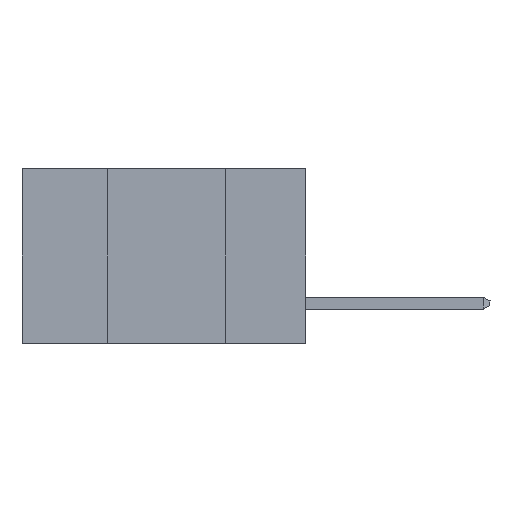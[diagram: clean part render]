
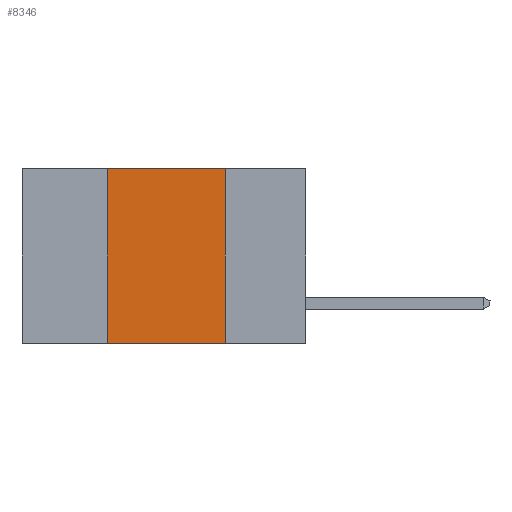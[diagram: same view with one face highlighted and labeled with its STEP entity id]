
A CAD part, left-side view. The second image highlights one B-rep face of the part: STEP entity #8346.
In plain terms, the highlighted planar face has unit normal (-1, 0, 0).
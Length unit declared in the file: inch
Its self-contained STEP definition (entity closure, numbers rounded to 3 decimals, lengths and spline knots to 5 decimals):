
#770 = VERTEX_POINT ( 'NONE', #22254 ) ;
#1752 = CARTESIAN_POINT ( 'NONE',  ( 0., 0.6, 0. ) ) ;
#2187 = VECTOR ( 'NONE', #15263, 39.37008 ) ;
#2382 = CARTESIAN_POINT ( 'NONE',  ( 0., 0.17, -0.37 ) ) ;
#3071 = EDGE_CURVE ( 'NONE', #770, #21164, #15459, .T. ) ;
#3164 = LINE ( 'NONE', #7046, #21861 ) ;
#3831 = ORIENTED_EDGE ( 'NONE', *, *, #11643, .F. ) ;
#4577 = AXIS2_PLACEMENT_3D ( 'NONE', #14930, #9579, #7918 ) ;
#7046 = CARTESIAN_POINT ( 'NONE',  ( 0., 0.42, 0. ) ) ;
#7918 = DIRECTION ( 'NONE',  ( 0., 0., -1. ) ) ;
#7944 = EDGE_LOOP ( 'NONE', ( #8499, #13922, #3831, #9128 ) ) ;
#8346 = ADVANCED_FACE ( 'NONE', ( #8992 ), #20260, .F. ) ;
#8499 = ORIENTED_EDGE ( 'NONE', *, *, #3071, .F. ) ;
#8992 = FACE_OUTER_BOUND ( 'NONE', #7944, .T. ) ;
#9128 = ORIENTED_EDGE ( 'NONE', *, *, #11788, .T. ) ;
#9579 = DIRECTION ( 'NONE',  ( 1., 0., 0. ) ) ;
#9797 = VERTEX_POINT ( 'NONE', #14344 ) ;
#10077 = CARTESIAN_POINT ( 'NONE',  ( 0., 0.17, 0. ) ) ;
#10163 = VECTOR ( 'NONE', #10986, 39.37008 ) ;
#10249 = VERTEX_POINT ( 'NONE', #18871 ) ;
#10726 = LINE ( 'NONE', #1752, #10163 ) ;
#10986 = DIRECTION ( 'NONE',  ( 0., -1., 0. ) ) ;
#11206 = CARTESIAN_POINT ( 'NONE',  ( 0., 0.6, -0.37 ) ) ;
#11643 = EDGE_CURVE ( 'NONE', #9797, #10249, #3164, .T. ) ;
#11788 = EDGE_CURVE ( 'NONE', #9797, #21164, #18172, .T. ) ;
#13922 = ORIENTED_EDGE ( 'NONE', *, *, #14867, .F. ) ;
#14343 = DIRECTION ( 'NONE',  ( 0., 0., 1. ) ) ;
#14344 = CARTESIAN_POINT ( 'NONE',  ( 0., 0.42, -0.37 ) ) ;
#14829 = DIRECTION ( 'NONE',  ( 0., -1., 0. ) ) ;
#14867 = EDGE_CURVE ( 'NONE', #10249, #770, #10726, .T. ) ;
#14930 = CARTESIAN_POINT ( 'NONE',  ( 0., 0.6, 0. ) ) ;
#15263 = DIRECTION ( 'NONE',  ( 0., 0., -1. ) ) ;
#15459 = LINE ( 'NONE', #10077, #2187 ) ;
#18172 = LINE ( 'NONE', #11206, #19890 ) ;
#18871 = CARTESIAN_POINT ( 'NONE',  ( 0., 0.42, 0. ) ) ;
#19890 = VECTOR ( 'NONE', #14829, 39.37008 ) ;
#20260 = PLANE ( 'NONE',  #4577 ) ;
#21164 = VERTEX_POINT ( 'NONE', #2382 ) ;
#21861 = VECTOR ( 'NONE', #14343, 39.37008 ) ;
#22254 = CARTESIAN_POINT ( 'NONE',  ( 0., 0.17, 0. ) ) ;
